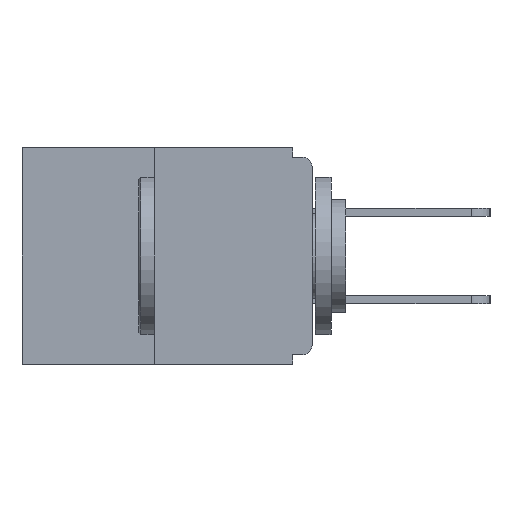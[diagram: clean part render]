
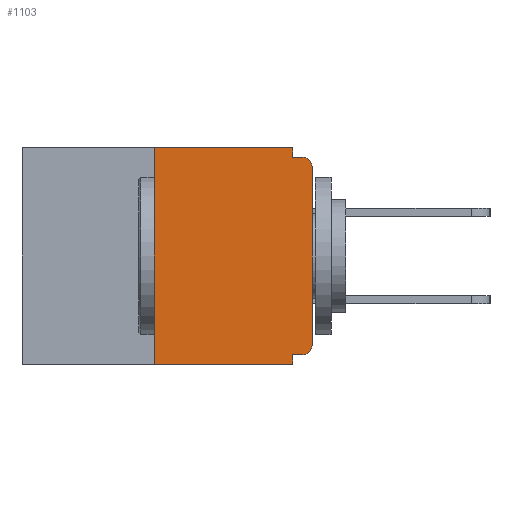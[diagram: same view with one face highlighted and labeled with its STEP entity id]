
A CAD part, left-side view. The second image highlights one B-rep face of the part: STEP entity #1103.
In plain terms, the highlighted planar face has unit normal (-1, 0, 0).
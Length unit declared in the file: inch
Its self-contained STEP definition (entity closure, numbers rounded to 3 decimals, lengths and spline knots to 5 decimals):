
#17 = LINE ( 'NONE', #25018, #21889 ) ;
#663 = LINE ( 'NONE', #23608, #7373 ) ;
#812 = EDGE_CURVE ( 'NONE', #17775, #22304, #10476, .T. ) ;
#1103 = ADVANCED_FACE ( 'NONE', ( #8313 ), #4526, .F. ) ;
#1345 = ORIENTED_EDGE ( 'NONE', *, *, #12000, .T. ) ;
#1483 = CARTESIAN_POINT ( 'NONE',  ( 0., 0., -0.015 ) ) ;
#1656 = ORIENTED_EDGE ( 'NONE', *, *, #5031, .F. ) ;
#1873 = DIRECTION ( 'NONE',  ( 0., 0., -1. ) ) ;
#2549 = CARTESIAN_POINT ( 'NONE',  ( 0., 0.25, 0. ) ) ;
#2731 = CARTESIAN_POINT ( 'NONE',  ( 0., 0.031, -0.343 ) ) ;
#2766 = DIRECTION ( 'NONE',  ( 0., 0., 1. ) ) ;
#3352 = CARTESIAN_POINT ( 'NONE',  ( 0., 0.031, 0. ) ) ;
#3759 = LINE ( 'NONE', #28373, #25299 ) ;
#4035 = VECTOR ( 'NONE', #7251, 39.37008 ) ;
#4173 = VERTEX_POINT ( 'NONE', #3352 ) ;
#4526 = PLANE ( 'NONE',  #9071 ) ;
#4579 = VERTEX_POINT ( 'NONE', #6011 ) ;
#4634 = VERTEX_POINT ( 'NONE', #27272 ) ;
#4906 = DIRECTION ( 'NONE',  ( 0., 0., -1. ) ) ;
#5031 = EDGE_CURVE ( 'NONE', #4634, #17476, #5384, .T. ) ;
#5289 = ORIENTED_EDGE ( 'NONE', *, *, #17782, .T. ) ;
#5384 = LINE ( 'NONE', #1483, #20131 ) ;
#5509 = DIRECTION ( 'NONE',  ( 0., 0., -1. ) ) ;
#5703 = ORIENTED_EDGE ( 'NONE', *, *, #13516, .F. ) ;
#5932 = CARTESIAN_POINT ( 'NONE',  ( 0., 0.015, -0.03 ) ) ;
#6011 = CARTESIAN_POINT ( 'NONE',  ( 0., 0.25, 0. ) ) ;
#6324 = VERTEX_POINT ( 'NONE', #13579 ) ;
#6335 = CARTESIAN_POINT ( 'NONE',  ( 0., 0.015, -0.015 ) ) ;
#6442 = DIRECTION ( 'NONE',  ( 0., 1., 0. ) ) ;
#6508 = CARTESIAN_POINT ( 'NONE',  ( 0., 0.25, -0.343 ) ) ;
#6705 = EDGE_CURVE ( 'NONE', #6324, #9592, #663, .T. ) ;
#7251 = DIRECTION ( 'NONE',  ( 0., -1., 0. ) ) ;
#7373 = VECTOR ( 'NONE', #5509, 39.37008 ) ;
#7525 = CARTESIAN_POINT ( 'NONE',  ( 0., 0.015, -0.313 ) ) ;
#8196 = VECTOR ( 'NONE', #2766, 39.37008 ) ;
#8313 = FACE_OUTER_BOUND ( 'NONE', #15342, .T. ) ;
#8891 = EDGE_CURVE ( 'NONE', #22304, #23295, #14033, .T. ) ;
#9071 = AXIS2_PLACEMENT_3D ( 'NONE', #20181, #22556, #1873 ) ;
#9592 = VERTEX_POINT ( 'NONE', #2731 ) ;
#9880 = DIRECTION ( 'NONE',  ( 0., -1., 0. ) ) ;
#9918 = VERTEX_POINT ( 'NONE', #6508 ) ;
#10476 = CIRCLE ( 'NONE', #22094, 0.015 ) ;
#10739 = LINE ( 'NONE', #18114, #4035 ) ;
#10749 = EDGE_CURVE ( 'NONE', #17775, #6324, #3759, .T. ) ;
#12000 = EDGE_CURVE ( 'NONE', #9918, #9592, #10739, .T. ) ;
#12252 = CARTESIAN_POINT ( 'NONE',  ( 0., 0., 0. ) ) ;
#12351 = VECTOR ( 'NONE', #14663, 39.37008 ) ;
#12667 = DIRECTION ( 'NONE',  ( 0., 0., -1. ) ) ;
#13516 = EDGE_CURVE ( 'NONE', #4173, #4634, #17, .T. ) ;
#13579 = CARTESIAN_POINT ( 'NONE',  ( 0., 0.031, -0.328 ) ) ;
#14033 = LINE ( 'NONE', #12252, #12351 ) ;
#14053 = CARTESIAN_POINT ( 'NONE',  ( 0., 0., -0.313 ) ) ;
#14663 = DIRECTION ( 'NONE',  ( 0., 0., 1. ) ) ;
#14999 = LINE ( 'NONE', #18924, #27436 ) ;
#15342 = EDGE_LOOP ( 'NONE', ( #22104, #23774, #1345, #19369, #17889, #25901, #19092, #5289, #1656, #5703 ) ) ;
#16354 = AXIS2_PLACEMENT_3D ( 'NONE', #5932, #26210, #12667 ) ;
#17476 = VERTEX_POINT ( 'NONE', #6335 ) ;
#17775 = VERTEX_POINT ( 'NONE', #19367 ) ;
#17782 = EDGE_CURVE ( 'NONE', #23295, #17476, #26324, .T. ) ;
#17889 = ORIENTED_EDGE ( 'NONE', *, *, #10749, .F. ) ;
#18114 = CARTESIAN_POINT ( 'NONE',  ( 0., 0.46, -0.343 ) ) ;
#18924 = CARTESIAN_POINT ( 'NONE',  ( 0., 0.46, 0. ) ) ;
#19092 = ORIENTED_EDGE ( 'NONE', *, *, #8891, .T. ) ;
#19357 = EDGE_CURVE ( 'NONE', #9918, #4579, #28350, .T. ) ;
#19367 = CARTESIAN_POINT ( 'NONE',  ( 0., 0.015, -0.328 ) ) ;
#19369 = ORIENTED_EDGE ( 'NONE', *, *, #6705, .F. ) ;
#20131 = VECTOR ( 'NONE', #28422, 39.37008 ) ;
#20181 = CARTESIAN_POINT ( 'NONE',  ( 0., 0.46, 0. ) ) ;
#21072 = CARTESIAN_POINT ( 'NONE',  ( 0., 0., -0.03 ) ) ;
#21889 = VECTOR ( 'NONE', #4906, 39.37008 ) ;
#22094 = AXIS2_PLACEMENT_3D ( 'NONE', #7525, #27751, #27852 ) ;
#22104 = ORIENTED_EDGE ( 'NONE', *, *, #26390, .F. ) ;
#22304 = VERTEX_POINT ( 'NONE', #14053 ) ;
#22556 = DIRECTION ( 'NONE',  ( 1., 0., 0. ) ) ;
#23295 = VERTEX_POINT ( 'NONE', #21072 ) ;
#23608 = CARTESIAN_POINT ( 'NONE',  ( 0., 0.031, -0.343 ) ) ;
#23774 = ORIENTED_EDGE ( 'NONE', *, *, #19357, .F. ) ;
#25018 = CARTESIAN_POINT ( 'NONE',  ( 0., 0.031, 0. ) ) ;
#25299 = VECTOR ( 'NONE', #6442, 39.37008 ) ;
#25901 = ORIENTED_EDGE ( 'NONE', *, *, #812, .T. ) ;
#26210 = DIRECTION ( 'NONE',  ( -1., 0., 0. ) ) ;
#26324 = CIRCLE ( 'NONE', #16354, 0.015 ) ;
#26390 = EDGE_CURVE ( 'NONE', #4579, #4173, #14999, .T. ) ;
#27272 = CARTESIAN_POINT ( 'NONE',  ( 0., 0.031, -0.015 ) ) ;
#27436 = VECTOR ( 'NONE', #9880, 39.37008 ) ;
#27751 = DIRECTION ( 'NONE',  ( -1., 0., 0. ) ) ;
#27852 = DIRECTION ( 'NONE',  ( 0., 0., -1. ) ) ;
#28350 = LINE ( 'NONE', #2549, #8196 ) ;
#28373 = CARTESIAN_POINT ( 'NONE',  ( 0., 0., -0.328 ) ) ;
#28422 = DIRECTION ( 'NONE',  ( 0., -1., 0. ) ) ;
